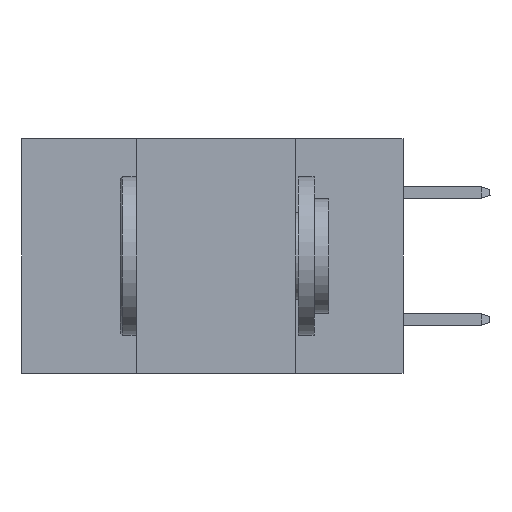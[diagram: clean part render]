
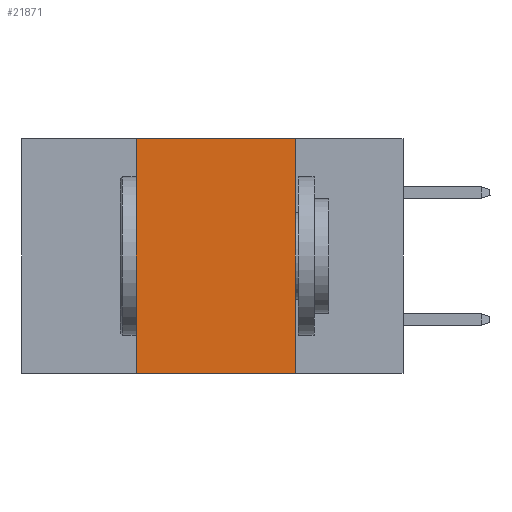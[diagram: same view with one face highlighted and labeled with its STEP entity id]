
A CAD part, left-side view. The second image highlights one B-rep face of the part: STEP entity #21871.
In plain terms, the highlighted planar face has unit normal (-1, 0, 0).
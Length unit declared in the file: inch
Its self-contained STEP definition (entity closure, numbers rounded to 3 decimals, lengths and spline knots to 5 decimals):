
#332 = ORIENTED_EDGE ( 'NONE', *, *, #30877, .F. ) ;
#884 = VERTEX_POINT ( 'NONE', #4672 ) ;
#1373 = DIRECTION ( 'NONE',  ( 0., 0., 1. ) ) ;
#1988 = CARTESIAN_POINT ( 'NONE',  ( 0., 0.17, 0. ) ) ;
#2481 = EDGE_CURVE ( 'NONE', #20497, #884, #6092, .T. ) ;
#3643 = EDGE_CURVE ( 'NONE', #884, #11566, #4370, .T. ) ;
#4370 = LINE ( 'NONE', #15223, #22863 ) ;
#4672 = CARTESIAN_POINT ( 'NONE',  ( 0., 0.42, 0. ) ) ;
#5188 = CARTESIAN_POINT ( 'NONE',  ( 0., 0.17, 0. ) ) ;
#6092 = LINE ( 'NONE', #11875, #26299 ) ;
#9098 = VECTOR ( 'NONE', #21962, 39.37008 ) ;
#9144 = DIRECTION ( 'NONE',  ( 1., 0., 0. ) ) ;
#10558 = ORIENTED_EDGE ( 'NONE', *, *, #2481, .F. ) ;
#11026 = CARTESIAN_POINT ( 'NONE',  ( 0., 0.17, -0.37 ) ) ;
#11279 = LINE ( 'NONE', #22325, #9098 ) ;
#11566 = VERTEX_POINT ( 'NONE', #5188 ) ;
#11875 = CARTESIAN_POINT ( 'NONE',  ( 0., 0.42, 0. ) ) ;
#12205 = CARTESIAN_POINT ( 'NONE',  ( 0., 0.6, 0. ) ) ;
#15223 = CARTESIAN_POINT ( 'NONE',  ( 0., 0.6, 0. ) ) ;
#15616 = AXIS2_PLACEMENT_3D ( 'NONE', #12205, #9144, #25633 ) ;
#17699 = EDGE_CURVE ( 'NONE', #20497, #35663, #11279, .T. ) ;
#20362 = FACE_OUTER_BOUND ( 'NONE', #20420, .T. ) ;
#20420 = EDGE_LOOP ( 'NONE', ( #332, #29129, #10558, #21818 ) ) ;
#20497 = VERTEX_POINT ( 'NONE', #34483 ) ;
#21818 = ORIENTED_EDGE ( 'NONE', *, *, #17699, .T. ) ;
#21871 = ADVANCED_FACE ( 'NONE', ( #20362 ), #26161, .F. ) ;
#21962 = DIRECTION ( 'NONE',  ( 0., -1., 0. ) ) ;
#22325 = CARTESIAN_POINT ( 'NONE',  ( 0., 0.6, -0.37 ) ) ;
#22863 = VECTOR ( 'NONE', #23372, 39.37008 ) ;
#23372 = DIRECTION ( 'NONE',  ( 0., -1., 0. ) ) ;
#24900 = VECTOR ( 'NONE', #29342, 39.37008 ) ;
#25633 = DIRECTION ( 'NONE',  ( 0., 0., -1. ) ) ;
#26161 = PLANE ( 'NONE',  #15616 ) ;
#26299 = VECTOR ( 'NONE', #1373, 39.37008 ) ;
#29129 = ORIENTED_EDGE ( 'NONE', *, *, #3643, .F. ) ;
#29342 = DIRECTION ( 'NONE',  ( 0., 0., -1. ) ) ;
#29515 = LINE ( 'NONE', #1988, #24900 ) ;
#30877 = EDGE_CURVE ( 'NONE', #11566, #35663, #29515, .T. ) ;
#34483 = CARTESIAN_POINT ( 'NONE',  ( 0., 0.42, -0.37 ) ) ;
#35663 = VERTEX_POINT ( 'NONE', #11026 ) ;
